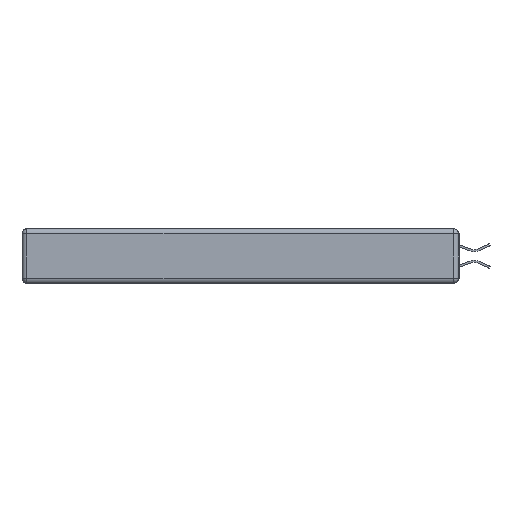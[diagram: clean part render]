
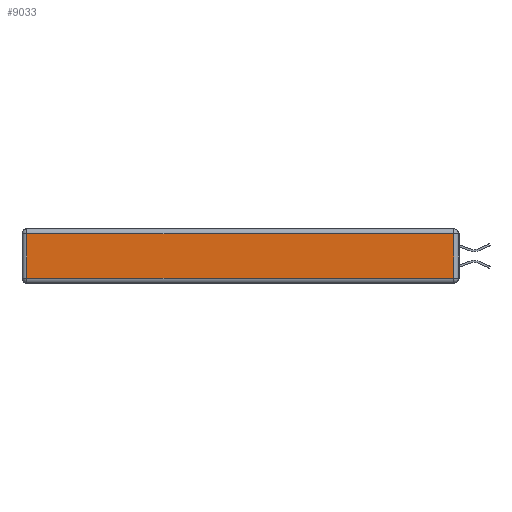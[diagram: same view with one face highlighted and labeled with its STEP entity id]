
A CAD part, left-side view. The second image highlights one B-rep face of the part: STEP entity #9033.
In plain terms, the highlighted planar face has unit normal (-1, 0, 0).
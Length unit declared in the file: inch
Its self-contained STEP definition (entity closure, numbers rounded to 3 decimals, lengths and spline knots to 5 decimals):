
#1697 = ORIENTED_EDGE ( 'NONE', *, *, #11774, .T. ) ;
#2249 = VERTEX_POINT ( 'NONE', #16584 ) ;
#2356 = VECTOR ( 'NONE', #3984, 39.37008 ) ;
#2498 = EDGE_CURVE ( 'NONE', #12899, #21009, #6769, .T. ) ;
#2698 = CARTESIAN_POINT ( 'NONE',  ( 0., 0.03, -0.313 ) ) ;
#3882 = CARTESIAN_POINT ( 'NONE',  ( 0., 2.75, -0.03 ) ) ;
#3984 = DIRECTION ( 'NONE',  ( 0., -1., 0. ) ) ;
#4079 = EDGE_CURVE ( 'NONE', #7193, #2249, #9292, .T. ) ;
#4807 = FACE_OUTER_BOUND ( 'NONE', #15490, .T. ) ;
#5509 = VECTOR ( 'NONE', #8850, 39.37008 ) ;
#5854 = ORIENTED_EDGE ( 'NONE', *, *, #4079, .T. ) ;
#5914 = CARTESIAN_POINT ( 'NONE',  ( 0., 0., -0.343 ) ) ;
#6026 = LINE ( 'NONE', #8635, #5509 ) ;
#6304 = CARTESIAN_POINT ( 'NONE',  ( 0., 0.03, -0.03 ) ) ;
#6769 = LINE ( 'NONE', #18859, #2356 ) ;
#7193 = VERTEX_POINT ( 'NONE', #6304 ) ;
#8635 = CARTESIAN_POINT ( 'NONE',  ( 0., 2.72, -0.343 ) ) ;
#8850 = DIRECTION ( 'NONE',  ( 0., 0., -1. ) ) ;
#9033 = ADVANCED_FACE ( 'NONE', ( #4807 ), #21022, .T. ) ;
#9096 = DIRECTION ( 'NONE',  ( 0., 0., 1. ) ) ;
#9292 = LINE ( 'NONE', #3882, #21558 ) ;
#10479 = CARTESIAN_POINT ( 'NONE',  ( 0., 0.03, -0.343 ) ) ;
#10977 = CARTESIAN_POINT ( 'NONE',  ( 0., 2.72, -0.313 ) ) ;
#11774 = EDGE_CURVE ( 'NONE', #2249, #12899, #6026, .T. ) ;
#12899 = VERTEX_POINT ( 'NONE', #10977 ) ;
#15187 = VECTOR ( 'NONE', #9096, 39.37008 ) ;
#15490 = EDGE_LOOP ( 'NONE', ( #21129, #16297, #5854, #1697 ) ) ;
#16297 = ORIENTED_EDGE ( 'NONE', *, *, #18733, .T. ) ;
#16584 = CARTESIAN_POINT ( 'NONE',  ( 0., 2.72, -0.03 ) ) ;
#17878 = AXIS2_PLACEMENT_3D ( 'NONE', #5914, #20836, #19299 ) ;
#18733 = EDGE_CURVE ( 'NONE', #21009, #7193, #21118, .T. ) ;
#18859 = CARTESIAN_POINT ( 'NONE',  ( 0., 0., -0.313 ) ) ;
#18982 = DIRECTION ( 'NONE',  ( 0., 1., 0. ) ) ;
#19299 = DIRECTION ( 'NONE',  ( 0., 0., 1. ) ) ;
#20836 = DIRECTION ( 'NONE',  ( -1., 0., 0. ) ) ;
#21009 = VERTEX_POINT ( 'NONE', #2698 ) ;
#21022 = PLANE ( 'NONE',  #17878 ) ;
#21118 = LINE ( 'NONE', #10479, #15187 ) ;
#21129 = ORIENTED_EDGE ( 'NONE', *, *, #2498, .T. ) ;
#21558 = VECTOR ( 'NONE', #18982, 39.37008 ) ;
